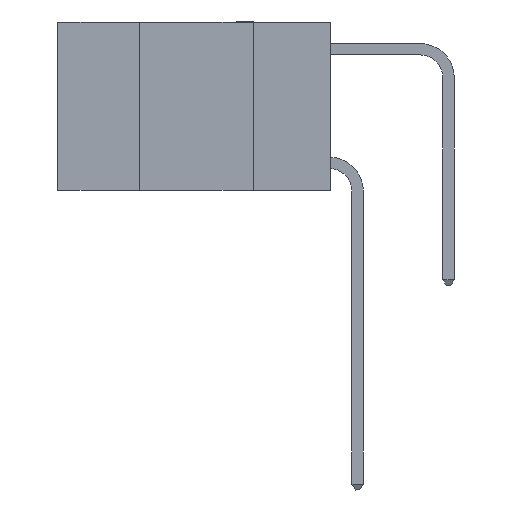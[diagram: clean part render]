
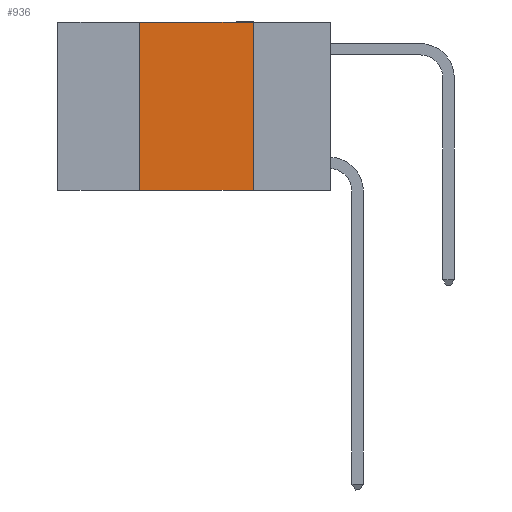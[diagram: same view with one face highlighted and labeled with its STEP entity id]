
A CAD part, left-side view. The second image highlights one B-rep face of the part: STEP entity #936.
In plain terms, the highlighted planar face has unit normal (-1, 0, 0).
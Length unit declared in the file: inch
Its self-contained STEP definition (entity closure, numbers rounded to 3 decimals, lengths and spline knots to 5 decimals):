
#237 = VERTEX_POINT ( 'NONE', #8750 ) ;
#363 = CARTESIAN_POINT ( 'NONE',  ( 0., 0.17, 0. ) ) ;
#936 = ADVANCED_FACE ( 'NONE', ( #7745 ), #11182, .F. ) ;
#963 = VECTOR ( 'NONE', #9611, 39.37008 ) ;
#1049 = CARTESIAN_POINT ( 'NONE',  ( 0., 0.42, 0. ) ) ;
#1129 = AXIS2_PLACEMENT_3D ( 'NONE', #9007, #4507, #7248 ) ;
#1167 = LINE ( 'NONE', #10371, #8492 ) ;
#1246 = VERTEX_POINT ( 'NONE', #6606 ) ;
#1307 = DIRECTION ( 'NONE',  ( 0., 0., -1. ) ) ;
#1630 = CARTESIAN_POINT ( 'NONE',  ( 0., 0.42, 0. ) ) ;
#2146 = VECTOR ( 'NONE', #12118, 39.37008 ) ;
#2725 = ORIENTED_EDGE ( 'NONE', *, *, #3014, .F. ) ;
#3014 = EDGE_CURVE ( 'NONE', #237, #9925, #4670, .T. ) ;
#3277 = ORIENTED_EDGE ( 'NONE', *, *, #6886, .F. ) ;
#3671 = DIRECTION ( 'NONE',  ( 0., -1., 0. ) ) ;
#4144 = VECTOR ( 'NONE', #1307, 39.37008 ) ;
#4155 = EDGE_LOOP ( 'NONE', ( #3277, #7437, #2725, #4755 ) ) ;
#4507 = DIRECTION ( 'NONE',  ( 1., 0., 0. ) ) ;
#4670 = LINE ( 'NONE', #1630, #2146 ) ;
#4755 = ORIENTED_EDGE ( 'NONE', *, *, #10311, .T. ) ;
#6606 = CARTESIAN_POINT ( 'NONE',  ( 0., 0.17, 0. ) ) ;
#6886 = EDGE_CURVE ( 'NONE', #1246, #7113, #12019, .T. ) ;
#7113 = VERTEX_POINT ( 'NONE', #8361 ) ;
#7186 = EDGE_CURVE ( 'NONE', #9925, #1246, #1167, .T. ) ;
#7248 = DIRECTION ( 'NONE',  ( 0., 0., -1. ) ) ;
#7437 = ORIENTED_EDGE ( 'NONE', *, *, #7186, .F. ) ;
#7745 = FACE_OUTER_BOUND ( 'NONE', #4155, .T. ) ;
#8361 = CARTESIAN_POINT ( 'NONE',  ( 0., 0.17, -0.37 ) ) ;
#8492 = VECTOR ( 'NONE', #3671, 39.37008 ) ;
#8646 = CARTESIAN_POINT ( 'NONE',  ( 0., 0.6, -0.37 ) ) ;
#8750 = CARTESIAN_POINT ( 'NONE',  ( 0., 0.42, -0.37 ) ) ;
#9007 = CARTESIAN_POINT ( 'NONE',  ( 0., 0.6, 0. ) ) ;
#9611 = DIRECTION ( 'NONE',  ( 0., -1., 0. ) ) ;
#9925 = VERTEX_POINT ( 'NONE', #1049 ) ;
#10311 = EDGE_CURVE ( 'NONE', #237, #7113, #11114, .T. ) ;
#10371 = CARTESIAN_POINT ( 'NONE',  ( 0., 0.6, 0. ) ) ;
#11114 = LINE ( 'NONE', #8646, #963 ) ;
#11182 = PLANE ( 'NONE',  #1129 ) ;
#12019 = LINE ( 'NONE', #363, #4144 ) ;
#12118 = DIRECTION ( 'NONE',  ( 0., 0., 1. ) ) ;
